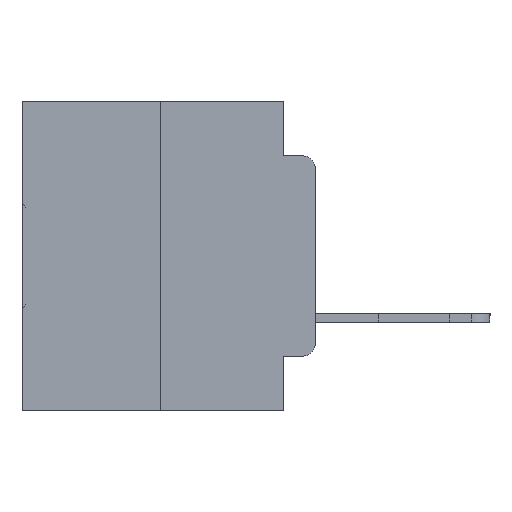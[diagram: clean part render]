
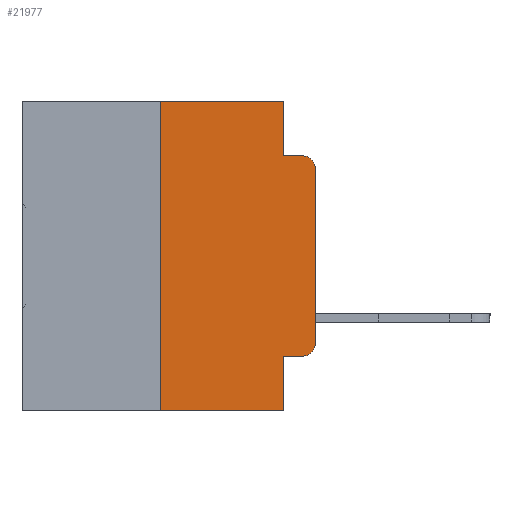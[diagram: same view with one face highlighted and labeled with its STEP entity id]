
A CAD part, left-side view. The second image highlights one B-rep face of the part: STEP entity #21977.
In plain terms, the highlighted planar face has unit normal (-1, 0, 0).
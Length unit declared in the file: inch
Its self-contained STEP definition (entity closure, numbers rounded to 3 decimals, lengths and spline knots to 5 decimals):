
#840 = ORIENTED_EDGE ( 'NONE', *, *, #22753, .F. ) ;
#1507 = CARTESIAN_POINT ( 'NONE',  ( 0., 0.051, -0.0885 ) ) ;
#1651 = VERTEX_POINT ( 'NONE', #15901 ) ;
#2174 = CARTESIAN_POINT ( 'NONE',  ( 0., 0.051, 0. ) ) ;
#2791 = EDGE_CURVE ( 'NONE', #12531, #32025, #14734, .T. ) ;
#2940 = VERTEX_POINT ( 'NONE', #8313 ) ;
#3061 = VERTEX_POINT ( 'NONE', #3663 ) ;
#3432 = CARTESIAN_POINT ( 'NONE',  ( 0., 0.25, 0. ) ) ;
#3663 = CARTESIAN_POINT ( 'NONE',  ( 0., 0.25, 0. ) ) ;
#3715 = DIRECTION ( 'NONE',  ( 1., 0., 0. ) ) ;
#3800 = AXIS2_PLACEMENT_3D ( 'NONE', #6026, #23691, #8682 ) ;
#4425 = VECTOR ( 'NONE', #13746, 39.37008 ) ;
#4668 = EDGE_CURVE ( 'NONE', #15940, #23892, #11722, .T. ) ;
#5223 = LINE ( 'NONE', #23563, #4425 ) ;
#5266 = ORIENTED_EDGE ( 'NONE', *, *, #2791, .F. ) ;
#5556 = VECTOR ( 'NONE', #11085, 39.37008 ) ;
#5567 = EDGE_CURVE ( 'NONE', #1651, #15887, #5223, .T. ) ;
#6026 = CARTESIAN_POINT ( 'NONE',  ( 0., 0.02, -0.3915 ) ) ;
#6213 = EDGE_CURVE ( 'NONE', #1651, #28334, #31390, .T. ) ;
#6412 = EDGE_CURVE ( 'NONE', #32025, #23892, #12881, .T. ) ;
#7626 = CARTESIAN_POINT ( 'NONE',  ( 0., 0.02, -0.0885 ) ) ;
#7627 = CARTESIAN_POINT ( 'NONE',  ( 0., 0.051, 0. ) ) ;
#8313 = CARTESIAN_POINT ( 'NONE',  ( 0., 0.25, -0.5 ) ) ;
#8682 = DIRECTION ( 'NONE',  ( 0., 0., -1. ) ) ;
#8831 = AXIS2_PLACEMENT_3D ( 'NONE', #18944, #3715, #21466 ) ;
#9069 = FACE_OUTER_BOUND ( 'NONE', #23389, .T. ) ;
#9353 = ORIENTED_EDGE ( 'NONE', *, *, #24312, .T. ) ;
#9797 = DIRECTION ( 'NONE',  ( 0., 0., 1. ) ) ;
#11085 = DIRECTION ( 'NONE',  ( 0., 0., -1. ) ) ;
#11537 = CARTESIAN_POINT ( 'NONE',  ( 0., 0.051, -0.0885 ) ) ;
#11722 = CIRCLE ( 'NONE', #18996, 0.02 ) ;
#11888 = DIRECTION ( 'NONE',  ( 0., -1., 0. ) ) ;
#12013 = CARTESIAN_POINT ( 'NONE',  ( 0., 0.473, 0. ) ) ;
#12060 = VECTOR ( 'NONE', #24244, 39.37008 ) ;
#12531 = VERTEX_POINT ( 'NONE', #2174 ) ;
#12709 = LINE ( 'NONE', #3432, #32363 ) ;
#12881 = LINE ( 'NONE', #1507, #12060 ) ;
#13746 = DIRECTION ( 'NONE',  ( 0., -1., 0. ) ) ;
#14225 = ORIENTED_EDGE ( 'NONE', *, *, #29110, .T. ) ;
#14503 = CARTESIAN_POINT ( 'NONE',  ( 0., 0.473, -0.5 ) ) ;
#14601 = ORIENTED_EDGE ( 'NONE', *, *, #31945, .F. ) ;
#14734 = LINE ( 'NONE', #7627, #27037 ) ;
#14909 = CARTESIAN_POINT ( 'NONE',  ( 0., 0.02, -0.1085 ) ) ;
#15205 = VECTOR ( 'NONE', #11888, 39.37008 ) ;
#15336 = VECTOR ( 'NONE', #9797, 39.37008 ) ;
#15887 = VERTEX_POINT ( 'NONE', #27599 ) ;
#15901 = CARTESIAN_POINT ( 'NONE',  ( 0., 0.051, -0.4115 ) ) ;
#15940 = VERTEX_POINT ( 'NONE', #22787 ) ;
#17174 = CARTESIAN_POINT ( 'NONE',  ( 0., 0., -0.3915 ) ) ;
#17388 = DIRECTION ( 'NONE',  ( 0., 0., -1. ) ) ;
#18008 = LINE ( 'NONE', #19781, #15336 ) ;
#18422 = ORIENTED_EDGE ( 'NONE', *, *, #18927, .T. ) ;
#18683 = DIRECTION ( 'NONE',  ( 0., 0., 1. ) ) ;
#18927 = EDGE_CURVE ( 'NONE', #32192, #15940, #18008, .T. ) ;
#18944 = CARTESIAN_POINT ( 'NONE',  ( 0., 0.473, 0. ) ) ;
#18996 = AXIS2_PLACEMENT_3D ( 'NONE', #14909, #32056, #17388 ) ;
#19781 = CARTESIAN_POINT ( 'NONE',  ( 0., 0., 0. ) ) ;
#19957 = ORIENTED_EDGE ( 'NONE', *, *, #4668, .T. ) ;
#21466 = DIRECTION ( 'NONE',  ( 0., 0., -1. ) ) ;
#21977 = ADVANCED_FACE ( 'NONE', ( #9069 ), #31086, .F. ) ;
#22753 = EDGE_CURVE ( 'NONE', #3061, #12531, #30304, .T. ) ;
#22787 = CARTESIAN_POINT ( 'NONE',  ( 0., 0., -0.1085 ) ) ;
#23026 = VECTOR ( 'NONE', #29321, 39.37008 ) ;
#23085 = ORIENTED_EDGE ( 'NONE', *, *, #6412, .F. ) ;
#23389 = EDGE_LOOP ( 'NONE', ( #18422, #19957, #23085, #5266, #840, #14601, #9353, #30745, #25767, #14225 ) ) ;
#23527 = CARTESIAN_POINT ( 'NONE',  ( 0., 0.051, 0. ) ) ;
#23563 = CARTESIAN_POINT ( 'NONE',  ( 0., 0.051, -0.4115 ) ) ;
#23691 = DIRECTION ( 'NONE',  ( -1., 0., 0. ) ) ;
#23780 = CIRCLE ( 'NONE', #3800, 0.02 ) ;
#23892 = VERTEX_POINT ( 'NONE', #7626 ) ;
#24244 = DIRECTION ( 'NONE',  ( 0., -1., 0. ) ) ;
#24312 = EDGE_CURVE ( 'NONE', #2940, #28334, #32448, .T. ) ;
#25767 = ORIENTED_EDGE ( 'NONE', *, *, #5567, .T. ) ;
#27037 = VECTOR ( 'NONE', #27655, 39.37008 ) ;
#27599 = CARTESIAN_POINT ( 'NONE',  ( 0., 0.02, -0.4115 ) ) ;
#27655 = DIRECTION ( 'NONE',  ( 0., 0., -1. ) ) ;
#28334 = VERTEX_POINT ( 'NONE', #29638 ) ;
#29110 = EDGE_CURVE ( 'NONE', #15887, #32192, #23780, .T. ) ;
#29321 = DIRECTION ( 'NONE',  ( 0., -1., 0. ) ) ;
#29638 = CARTESIAN_POINT ( 'NONE',  ( 0., 0.051, -0.5 ) ) ;
#30304 = LINE ( 'NONE', #12013, #23026 ) ;
#30745 = ORIENTED_EDGE ( 'NONE', *, *, #6213, .F. ) ;
#31086 = PLANE ( 'NONE',  #8831 ) ;
#31390 = LINE ( 'NONE', #23527, #5556 ) ;
#31945 = EDGE_CURVE ( 'NONE', #2940, #3061, #12709, .T. ) ;
#32025 = VERTEX_POINT ( 'NONE', #11537 ) ;
#32056 = DIRECTION ( 'NONE',  ( -1., 0., 0. ) ) ;
#32192 = VERTEX_POINT ( 'NONE', #17174 ) ;
#32363 = VECTOR ( 'NONE', #18683, 39.37008 ) ;
#32448 = LINE ( 'NONE', #14503, #15205 ) ;
